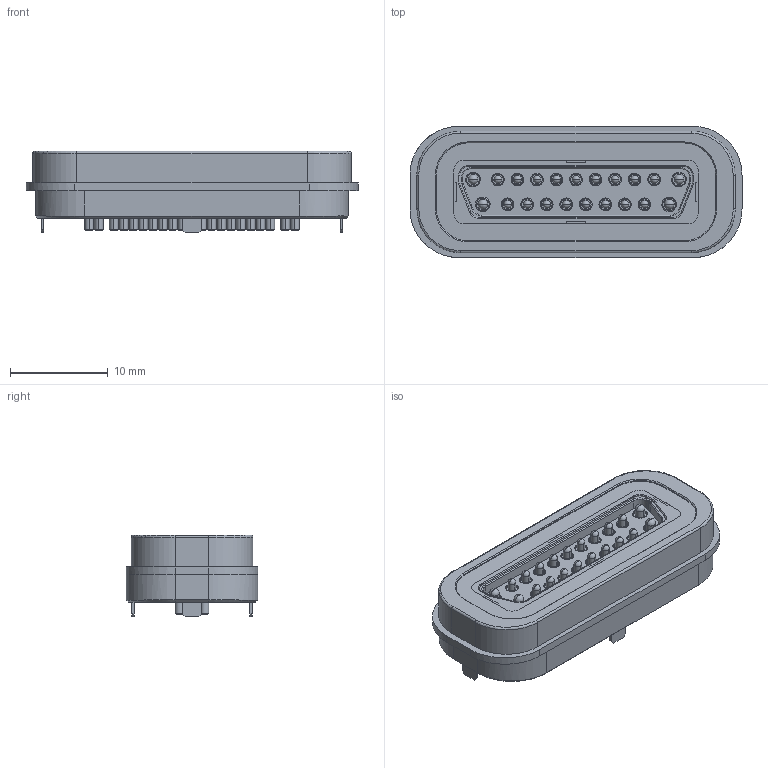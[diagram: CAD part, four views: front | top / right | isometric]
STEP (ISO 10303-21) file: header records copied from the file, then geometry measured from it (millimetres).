
FILE_DESCRIPTION (( 'STEP AP214' ), '1' );
FILE_NAME ('685A2131260111E.STEP', '2023-04-25T17:26:10', ( '' ), ( '' ), 'SwSTEP 2.0', 'SolidWorks 2020', '' );
FILE_SCHEMA (( 'AUTOMOTIVE_DESIGN' ));
Length unit declared in the file: millimetre
Products named in the file (1): 685A2131260111E
Bounding box: 33.98 x 13.44 x 8.35 mm (x, y, z)
Surface area: 5901.5 mm2
Topology: 7 solids, 7 shells, 1308 faces, 3038 edges, 1874 vertices
Faces by surface type: cylinder 540, plane 448, torus 132, cone 104, sphere 84
Entity records: 60276 total; most frequent: CARTESIAN_POINT 22654, ORIENTED_EDGE 5824, EDGE_CURVE 2912, B_SPLINE_CURVE_WITH_KNOTS 2796, DIRECTION 2764, VERTEX_POINT 1832, EDGE_LOOP 1532, AXIS2_PLACEMENT_3D 1339
